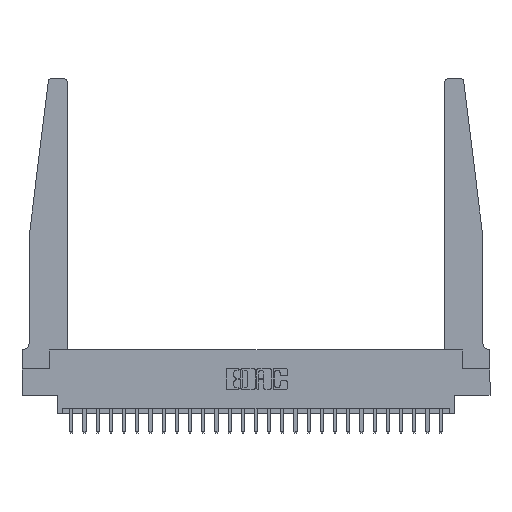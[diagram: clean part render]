
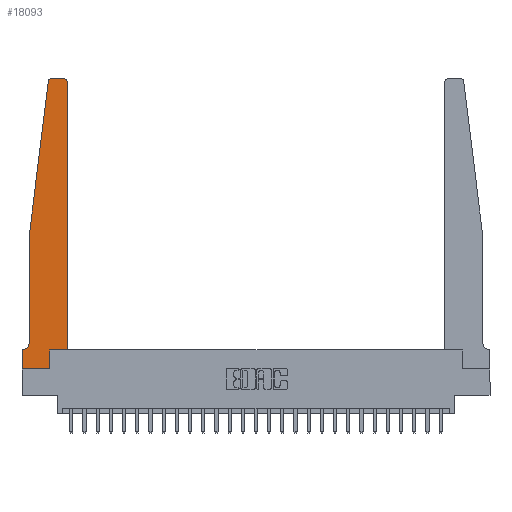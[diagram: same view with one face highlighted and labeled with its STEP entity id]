
A CAD part, top view. The second image highlights one B-rep face of the part: STEP entity #18093.
In plain terms, the highlighted planar face has unit normal (0, 0, 1).
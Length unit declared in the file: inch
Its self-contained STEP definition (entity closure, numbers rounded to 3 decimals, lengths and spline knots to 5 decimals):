
#678 = EDGE_CURVE ( 'NONE', #2742, #7026, #10432, .T. ) ;
#912 = EDGE_CURVE ( 'NONE', #11407, #1353, #10060, .T. ) ;
#1353 = VERTEX_POINT ( 'NONE', #22212 ) ;
#1390 = CARTESIAN_POINT ( 'NONE',  ( 0.425, 0.18, 0.37 ) ) ;
#1617 = DIRECTION ( 'NONE',  ( 0., -1., 0. ) ) ;
#1653 = DIRECTION ( 'NONE',  ( 0., 0., 1. ) ) ;
#1791 = LINE ( 'NONE', #11609, #20505 ) ;
#2274 = VECTOR ( 'NONE', #11815, 39.37008 ) ;
#2742 = VERTEX_POINT ( 'NONE', #2912 ) ;
#2912 = CARTESIAN_POINT ( 'NONE',  ( 0.065, 0.2375, 0.37 ) ) ;
#3081 = VERTEX_POINT ( 'NONE', #21035 ) ;
#3264 = CARTESIAN_POINT ( 'NONE',  ( 0.25, 2.75, 0.37 ) ) ;
#3692 = CARTESIAN_POINT ( 'NONE',  ( 0.425, 0.18, 0.37 ) ) ;
#3823 = EDGE_CURVE ( 'NONE', #19775, #18406, #25762, .T. ) ;
#5007 = DIRECTION ( 'NONE',  ( 0., 0., -1. ) ) ;
#5145 = ORIENTED_EDGE ( 'NONE', *, *, #11448, .T. ) ;
#5873 = CARTESIAN_POINT ( 'NONE',  ( 0.395, 2.75, 0.37 ) ) ;
#6315 = VECTOR ( 'NONE', #21359, 39.37008 ) ;
#6485 = LINE ( 'NONE', #20686, #6315 ) ;
#6561 = ORIENTED_EDGE ( 'NONE', *, *, #20214, .T. ) ;
#6959 = AXIS2_PLACEMENT_3D ( 'NONE', #12647, #18742, #16611 ) ;
#7026 = VERTEX_POINT ( 'NONE', #24310 ) ;
#7371 = ORIENTED_EDGE ( 'NONE', *, *, #12878, .T. ) ;
#8214 = CIRCLE ( 'NONE', #16725, 0.03 ) ;
#8605 = DIRECTION ( 'NONE',  ( 1., 0., 0. ) ) ;
#8867 = CARTESIAN_POINT ( 'NONE',  ( 0., 0., 0.37 ) ) ;
#9195 = CARTESIAN_POINT ( 'NONE',  ( 0.425, 2.72, 0.37 ) ) ;
#10060 = LINE ( 'NONE', #18170, #25227 ) ;
#10113 = CARTESIAN_POINT ( 'NONE',  ( 0.065, 1.25, 0.37 ) ) ;
#10127 = DIRECTION ( 'NONE',  ( 0., 1., 0. ) ) ;
#10217 = EDGE_CURVE ( 'NONE', #1353, #3081, #1791, .T. ) ;
#10238 = ORIENTED_EDGE ( 'NONE', *, *, #912, .T. ) ;
#10432 = CIRCLE ( 'NONE', #25192, 0.05 ) ;
#11407 = VERTEX_POINT ( 'NONE', #8867 ) ;
#11448 = EDGE_CURVE ( 'NONE', #16438, #16172, #8214, .T. ) ;
#11609 = CARTESIAN_POINT ( 'NONE',  ( 0.2605, 0.18, 0.37 ) ) ;
#11699 = LINE ( 'NONE', #19789, #12162 ) ;
#11815 = DIRECTION ( 'NONE',  ( 1., 0., 0. ) ) ;
#11915 = ORIENTED_EDGE ( 'NONE', *, *, #22354, .T. ) ;
#12162 = VECTOR ( 'NONE', #1617, 39.37008 ) ;
#12647 = CARTESIAN_POINT ( 'NONE',  ( 0., 0.1875, 0.37 ) ) ;
#12739 = DIRECTION ( 'NONE',  ( 0., 0., 1. ) ) ;
#12878 = EDGE_CURVE ( 'NONE', #3081, #19772, #23816, .T. ) ;
#13052 = PLANE ( 'NONE',  #6959 ) ;
#13602 = VECTOR ( 'NONE', #14446, 39.37008 ) ;
#14058 = DIRECTION ( 'NONE',  ( 1., 0., 0. ) ) ;
#14085 = ORIENTED_EDGE ( 'NONE', *, *, #3823, .T. ) ;
#14446 = DIRECTION ( 'NONE',  ( 0., -1., 0. ) ) ;
#14516 = FACE_OUTER_BOUND ( 'NONE', #25622, .T. ) ;
#14577 = DIRECTION ( 'NONE',  ( -0.122, -0.992, 0. ) ) ;
#14622 = CARTESIAN_POINT ( 'NONE',  ( 0.395, 2.72, 0.37 ) ) ;
#14712 = LINE ( 'NONE', #24434, #13602 ) ;
#14834 = CARTESIAN_POINT ( 'NONE',  ( 0.065, 1.25, 0.37 ) ) ;
#14862 = EDGE_CURVE ( 'NONE', #16172, #19775, #21426, .T. ) ;
#15487 = ORIENTED_EDGE ( 'NONE', *, *, #18364, .T. ) ;
#15642 = ORIENTED_EDGE ( 'NONE', *, *, #678, .T. ) ;
#15687 = VERTEX_POINT ( 'NONE', #17895 ) ;
#16028 = EDGE_CURVE ( 'NONE', #18406, #16713, #19056, .T. ) ;
#16160 = ORIENTED_EDGE ( 'NONE', *, *, #25026, .T. ) ;
#16172 = VERTEX_POINT ( 'NONE', #5873 ) ;
#16438 = VERTEX_POINT ( 'NONE', #9195 ) ;
#16611 = DIRECTION ( 'NONE',  ( 1., 0., 0. ) ) ;
#16713 = VERTEX_POINT ( 'NONE', #10113 ) ;
#16725 = AXIS2_PLACEMENT_3D ( 'NONE', #14622, #12739, #8605 ) ;
#16848 = ORIENTED_EDGE ( 'NONE', *, *, #14862, .T. ) ;
#17031 = LINE ( 'NONE', #19153, #22536 ) ;
#17126 = DIRECTION ( 'NONE',  ( -1., 0., 0. ) ) ;
#17436 = CARTESIAN_POINT ( 'NONE',  ( 0.27653, 2.75, 0.37 ) ) ;
#17841 = DIRECTION ( 'NONE',  ( 1., 0., 0. ) ) ;
#17895 = CARTESIAN_POINT ( 'NONE',  ( 0., 0.1875, 0.37 ) ) ;
#18093 = ADVANCED_FACE ( 'NONE', ( #14516 ), #13052, .T. ) ;
#18170 = CARTESIAN_POINT ( 'NONE',  ( 0., 0., 0.37 ) ) ;
#18364 = EDGE_CURVE ( 'NONE', #15687, #11407, #11699, .T. ) ;
#18406 = VERTEX_POINT ( 'NONE', #22269 ) ;
#18492 = CARTESIAN_POINT ( 'NONE',  ( 0.015, 0.2375, 0.37 ) ) ;
#18742 = DIRECTION ( 'NONE',  ( 0., 0., 1. ) ) ;
#18889 = DIRECTION ( 'NONE',  ( -1., 0., 0. ) ) ;
#19056 = LINE ( 'NONE', #14834, #23755 ) ;
#19153 = CARTESIAN_POINT ( 'NONE',  ( 0.065, 0.1875, 0.37 ) ) ;
#19457 = DIRECTION ( 'NONE',  ( -1., 0., 0. ) ) ;
#19772 = VERTEX_POINT ( 'NONE', #1390 ) ;
#19775 = VERTEX_POINT ( 'NONE', #17436 ) ;
#19789 = CARTESIAN_POINT ( 'NONE',  ( 0., 0., 0.37 ) ) ;
#20214 = EDGE_CURVE ( 'NONE', #19772, #16438, #6485, .T. ) ;
#20505 = VECTOR ( 'NONE', #10127, 39.37008 ) ;
#20686 = CARTESIAN_POINT ( 'NONE',  ( 0.425, 0.18, 0.37 ) ) ;
#20692 = AXIS2_PLACEMENT_3D ( 'NONE', #23234, #1653, #17841 ) ;
#21035 = CARTESIAN_POINT ( 'NONE',  ( 0.2605, 0.18, 0.37 ) ) ;
#21359 = DIRECTION ( 'NONE',  ( 0., 1., 0. ) ) ;
#21426 = LINE ( 'NONE', #3264, #23280 ) ;
#22212 = CARTESIAN_POINT ( 'NONE',  ( 0.2605, 0., 0.37 ) ) ;
#22269 = CARTESIAN_POINT ( 'NONE',  ( 0.24675, 2.72367, 0.37 ) ) ;
#22354 = EDGE_CURVE ( 'NONE', #16713, #2742, #14712, .T. ) ;
#22536 = VECTOR ( 'NONE', #18889, 39.37008 ) ;
#23234 = CARTESIAN_POINT ( 'NONE',  ( 0.27653, 2.72, 0.37 ) ) ;
#23280 = VECTOR ( 'NONE', #19457, 39.37008 ) ;
#23383 = ORIENTED_EDGE ( 'NONE', *, *, #10217, .T. ) ;
#23755 = VECTOR ( 'NONE', #14577, 39.37008 ) ;
#23816 = LINE ( 'NONE', #3692, #2274 ) ;
#24310 = CARTESIAN_POINT ( 'NONE',  ( 0.015, 0.1875, 0.37 ) ) ;
#24434 = CARTESIAN_POINT ( 'NONE',  ( 0.065, 1.25, 0.37 ) ) ;
#25026 = EDGE_CURVE ( 'NONE', #7026, #15687, #17031, .T. ) ;
#25192 = AXIS2_PLACEMENT_3D ( 'NONE', #18492, #5007, #17126 ) ;
#25227 = VECTOR ( 'NONE', #14058, 39.37008 ) ;
#25392 = ORIENTED_EDGE ( 'NONE', *, *, #16028, .T. ) ;
#25622 = EDGE_LOOP ( 'NONE', ( #16848, #14085, #25392, #11915, #15642, #16160, #15487, #10238, #23383, #7371, #6561, #5145 ) ) ;
#25762 = CIRCLE ( 'NONE', #20692, 0.03 ) ;
